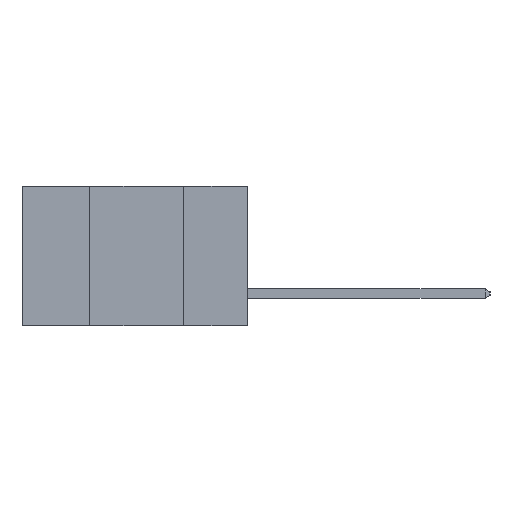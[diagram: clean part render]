
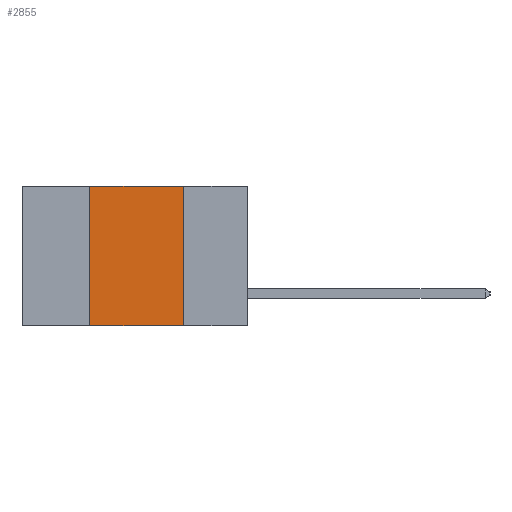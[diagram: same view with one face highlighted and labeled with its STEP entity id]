
A CAD part, left-side view. The second image highlights one B-rep face of the part: STEP entity #2855.
In plain terms, the highlighted planar face has unit normal (-1, 0, 0).
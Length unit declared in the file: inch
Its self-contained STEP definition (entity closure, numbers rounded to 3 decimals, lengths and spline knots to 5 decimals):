
#47 = ORIENTED_EDGE ( 'NONE', *, *, #1912, .F. ) ;
#251 = LINE ( 'NONE', #13248, #16291 ) ;
#1002 = EDGE_CURVE ( 'NONE', #10655, #7617, #251, .T. ) ;
#1912 = EDGE_CURVE ( 'NONE', #7617, #15087, #13416, .T. ) ;
#2217 = ORIENTED_EDGE ( 'NONE', *, *, #1002, .F. ) ;
#2340 = AXIS2_PLACEMENT_3D ( 'NONE', #3228, #2994, #3012 ) ;
#2820 = DIRECTION ( 'NONE',  ( 0., -1., 0. ) ) ;
#2855 = ADVANCED_FACE ( 'NONE', ( #15582 ), #3077, .F. ) ;
#2994 = DIRECTION ( 'NONE',  ( 1., 0., 0. ) ) ;
#3012 = DIRECTION ( 'NONE',  ( 0., 0., -1. ) ) ;
#3077 = PLANE ( 'NONE',  #2340 ) ;
#3228 = CARTESIAN_POINT ( 'NONE',  ( 0., 0.6, 0. ) ) ;
#3635 = EDGE_CURVE ( 'NONE', #15087, #13362, #9001, .T. ) ;
#3748 = ORIENTED_EDGE ( 'NONE', *, *, #3635, .F. ) ;
#4062 = CARTESIAN_POINT ( 'NONE',  ( 0., 0.6, -0.37 ) ) ;
#4324 = DIRECTION ( 'NONE',  ( 0., -1., 0. ) ) ;
#4379 = CARTESIAN_POINT ( 'NONE',  ( 0., 0.6, 0. ) ) ;
#7617 = VERTEX_POINT ( 'NONE', #13453 ) ;
#8646 = CARTESIAN_POINT ( 'NONE',  ( 0., 0.17, 0. ) ) ;
#9001 = LINE ( 'NONE', #10280, #11939 ) ;
#9726 = ORIENTED_EDGE ( 'NONE', *, *, #14103, .T. ) ;
#9774 = VECTOR ( 'NONE', #2820, 39.37008 ) ;
#10110 = DIRECTION ( 'NONE',  ( 0., 0., -1. ) ) ;
#10179 = VECTOR ( 'NONE', #4324, 39.37008 ) ;
#10280 = CARTESIAN_POINT ( 'NONE',  ( 0., 0.17, -0.37 ) ) ;
#10428 = CARTESIAN_POINT ( 'NONE',  ( 0., 0.42, -0.37 ) ) ;
#10655 = VERTEX_POINT ( 'NONE', #10428 ) ;
#11575 = CARTESIAN_POINT ( 'NONE',  ( 0., 0.17, -0.37 ) ) ;
#11939 = VECTOR ( 'NONE', #10110, 39.37008 ) ;
#12169 = EDGE_LOOP ( 'NONE', ( #3748, #47, #2217, #9726 ) ) ;
#13166 = DIRECTION ( 'NONE',  ( 0., 0., 1. ) ) ;
#13248 = CARTESIAN_POINT ( 'NONE',  ( 0., 0.42, -0.37 ) ) ;
#13362 = VERTEX_POINT ( 'NONE', #11575 ) ;
#13416 = LINE ( 'NONE', #4379, #10179 ) ;
#13453 = CARTESIAN_POINT ( 'NONE',  ( 0., 0.42, 0. ) ) ;
#13782 = LINE ( 'NONE', #4062, #9774 ) ;
#14103 = EDGE_CURVE ( 'NONE', #10655, #13362, #13782, .T. ) ;
#15087 = VERTEX_POINT ( 'NONE', #8646 ) ;
#15582 = FACE_OUTER_BOUND ( 'NONE', #12169, .T. ) ;
#16291 = VECTOR ( 'NONE', #13166, 39.37008 ) ;
